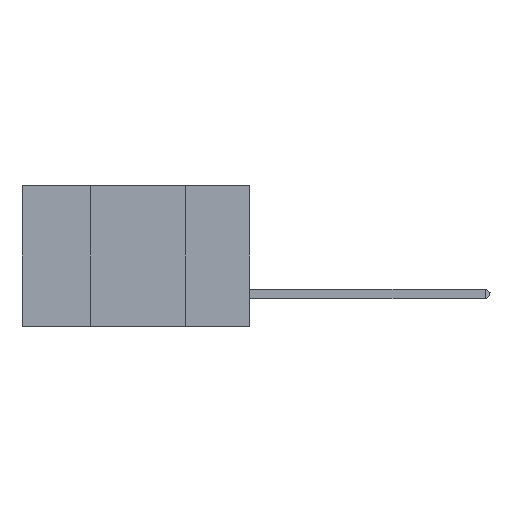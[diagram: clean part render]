
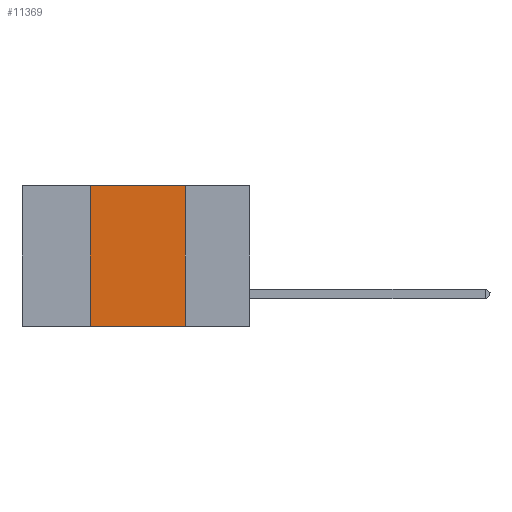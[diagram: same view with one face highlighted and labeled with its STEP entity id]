
A CAD part, left-side view. The second image highlights one B-rep face of the part: STEP entity #11369.
In plain terms, the highlighted planar face has unit normal (-1, 0, 0).
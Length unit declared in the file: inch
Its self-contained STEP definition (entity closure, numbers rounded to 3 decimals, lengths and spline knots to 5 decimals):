
#256 = DIRECTION ( 'NONE',  ( 0., 0., 1. ) ) ;
#2421 = VECTOR ( 'NONE', #256, 39.37008 ) ;
#3822 = LINE ( 'NONE', #11133, #18702 ) ;
#5069 = EDGE_CURVE ( 'NONE', #10139, #11067, #18778, .T. ) ;
#5223 = CARTESIAN_POINT ( 'NONE',  ( 0., 0.6, 0. ) ) ;
#5822 = DIRECTION ( 'NONE',  ( 0., -1., 0. ) ) ;
#7434 = DIRECTION ( 'NONE',  ( 0., 0., -1. ) ) ;
#7541 = CARTESIAN_POINT ( 'NONE',  ( 0., 0.42, -0.37 ) ) ;
#7568 = CARTESIAN_POINT ( 'NONE',  ( 0., 0.17, 0. ) ) ;
#8017 = ORIENTED_EDGE ( 'NONE', *, *, #13767, .F. ) ;
#8293 = FACE_OUTER_BOUND ( 'NONE', #19974, .T. ) ;
#9311 = CARTESIAN_POINT ( 'NONE',  ( 0., 0.42, 0. ) ) ;
#9538 = CARTESIAN_POINT ( 'NONE',  ( 0., 0.17, 0. ) ) ;
#9661 = ORIENTED_EDGE ( 'NONE', *, *, #5069, .T. ) ;
#10139 = VERTEX_POINT ( 'NONE', #7541 ) ;
#10916 = CARTESIAN_POINT ( 'NONE',  ( 0., 0.17, -0.37 ) ) ;
#11067 = VERTEX_POINT ( 'NONE', #10916 ) ;
#11133 = CARTESIAN_POINT ( 'NONE',  ( 0., 0.6, 0. ) ) ;
#11369 = ADVANCED_FACE ( 'NONE', ( #8293 ), #18491, .F. ) ;
#12184 = AXIS2_PLACEMENT_3D ( 'NONE', #5223, #20709, #7434 ) ;
#13767 = EDGE_CURVE ( 'NONE', #15437, #11067, #14948, .T. ) ;
#14210 = LINE ( 'NONE', #9311, #2421 ) ;
#14948 = LINE ( 'NONE', #7568, #22271 ) ;
#15437 = VERTEX_POINT ( 'NONE', #9538 ) ;
#15672 = DIRECTION ( 'NONE',  ( 0., -1., 0. ) ) ;
#17181 = ORIENTED_EDGE ( 'NONE', *, *, #25164, .F. ) ;
#18491 = PLANE ( 'NONE',  #12184 ) ;
#18702 = VECTOR ( 'NONE', #15672, 39.37008 ) ;
#18778 = LINE ( 'NONE', #19078, #20146 ) ;
#19078 = CARTESIAN_POINT ( 'NONE',  ( 0., 0.6, -0.37 ) ) ;
#19974 = EDGE_LOOP ( 'NONE', ( #8017, #17181, #27569, #9661 ) ) ;
#20146 = VECTOR ( 'NONE', #5822, 39.37008 ) ;
#20177 = EDGE_CURVE ( 'NONE', #10139, #27458, #14210, .T. ) ;
#20709 = DIRECTION ( 'NONE',  ( 1., 0., 0. ) ) ;
#22271 = VECTOR ( 'NONE', #27488, 39.37008 ) ;
#25039 = CARTESIAN_POINT ( 'NONE',  ( 0., 0.42, 0. ) ) ;
#25164 = EDGE_CURVE ( 'NONE', #27458, #15437, #3822, .T. ) ;
#27458 = VERTEX_POINT ( 'NONE', #25039 ) ;
#27488 = DIRECTION ( 'NONE',  ( 0., 0., -1. ) ) ;
#27569 = ORIENTED_EDGE ( 'NONE', *, *, #20177, .F. ) ;
